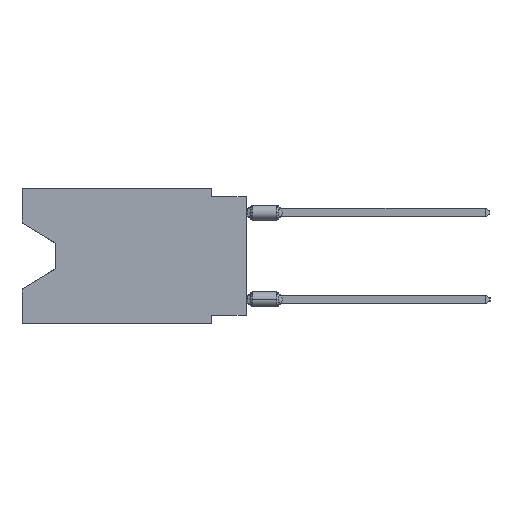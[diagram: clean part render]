
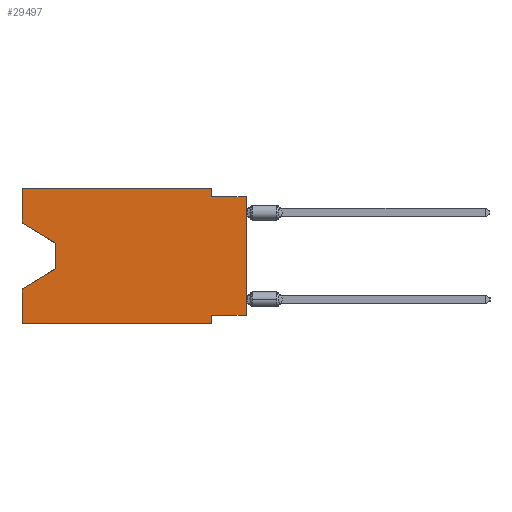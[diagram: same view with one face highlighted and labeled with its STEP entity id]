
A CAD part, left-side view. The second image highlights one B-rep face of the part: STEP entity #29497.
In plain terms, the highlighted planar face has unit normal (-1, 0, 0).
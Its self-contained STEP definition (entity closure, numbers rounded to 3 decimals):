
#1516 = CARTESIAN_POINT ( 'NONE',  ( 0., 16.383, 0. ) ) ;
#2131 = EDGE_CURVE ( 'NONE', #55517, #2793, #15696, .T. ) ;
#2134 = DIRECTION ( 'NONE',  ( 1., 0., 0. ) ) ;
#2793 = VERTEX_POINT ( 'NONE', #14090 ) ;
#3090 = CARTESIAN_POINT ( 'NONE',  ( 0., 0., -9.271 ) ) ;
#4744 = VERTEX_POINT ( 'NONE', #49859 ) ;
#5263 = VECTOR ( 'NONE', #22718, 1000. ) ;
#5686 = CARTESIAN_POINT ( 'NONE',  ( 0., 16.383, -9.906 ) ) ;
#6426 = FACE_OUTER_BOUND ( 'NONE', #46369, .T. ) ;
#6665 = EDGE_CURVE ( 'NONE', #55517, #16971, #51575, .T. ) ;
#7134 = VECTOR ( 'NONE', #56173, 1000. ) ;
#7454 = DIRECTION ( 'NONE',  ( 0., -1., 0. ) ) ;
#8672 = ORIENTED_EDGE ( 'NONE', *, *, #14410, .T. ) ;
#9556 = LINE ( 'NONE', #57363, #22292 ) ;
#12483 = VECTOR ( 'NONE', #55267, 1000. ) ;
#12492 = VECTOR ( 'NONE', #58864, 1000. ) ;
#12715 = VECTOR ( 'NONE', #55784, 1000. ) ;
#13063 = VECTOR ( 'NONE', #7454, 1000. ) ;
#13219 = CARTESIAN_POINT ( 'NONE',  ( 0., 13.97, -5.893 ) ) ;
#14090 = CARTESIAN_POINT ( 'NONE',  ( 0., 0., -0.635 ) ) ;
#14141 = DIRECTION ( 'NONE',  ( 0., 0.855, -0.519 ) ) ;
#14410 = EDGE_CURVE ( 'NONE', #4744, #47145, #36544, .T. ) ;
#15131 = CARTESIAN_POINT ( 'NONE',  ( 0., 2.54, -9.271 ) ) ;
#15696 = LINE ( 'NONE', #25502, #26946 ) ;
#16569 = VERTEX_POINT ( 'NONE', #28722 ) ;
#16971 = VERTEX_POINT ( 'NONE', #15131 ) ;
#17070 = CARTESIAN_POINT ( 'NONE',  ( 0., 16.383, 0. ) ) ;
#18372 = LINE ( 'NONE', #38292, #12715 ) ;
#19818 = EDGE_CURVE ( 'NONE', #55178, #34603, #37780, .T. ) ;
#20383 = DIRECTION ( 'NONE',  ( 0., -1., 0. ) ) ;
#20387 = ORIENTED_EDGE ( 'NONE', *, *, #24334, .T. ) ;
#20708 = VERTEX_POINT ( 'NONE', #33356 ) ;
#22292 = VECTOR ( 'NONE', #46996, 1000. ) ;
#22568 = CARTESIAN_POINT ( 'NONE',  ( 0., 2.54, 0. ) ) ;
#22718 = DIRECTION ( 'NONE',  ( 0., 0., 1. ) ) ;
#23934 = VECTOR ( 'NONE', #50823, 1000. ) ;
#24334 = EDGE_CURVE ( 'NONE', #34603, #4744, #9556, .T. ) ;
#24464 = CARTESIAN_POINT ( 'NONE',  ( 0., 16.383, -7.36 ) ) ;
#25063 = EDGE_CURVE ( 'NONE', #16569, #52150, #40426, .T. ) ;
#25502 = CARTESIAN_POINT ( 'NONE',  ( 0., 0., 0. ) ) ;
#25751 = CARTESIAN_POINT ( 'NONE',  ( 0., 2.54, 0. ) ) ;
#25879 = CARTESIAN_POINT ( 'NONE',  ( 0., 0., -0.635 ) ) ;
#26343 = EDGE_CURVE ( 'NONE', #35759, #20708, #35380, .T. ) ;
#26350 = ORIENTED_EDGE ( 'NONE', *, *, #44502, .F. ) ;
#26946 = VECTOR ( 'NONE', #39613, 1000. ) ;
#27565 = VERTEX_POINT ( 'NONE', #36009 ) ;
#27992 = EDGE_CURVE ( 'NONE', #55178, #16569, #49739, .T. ) ;
#28722 = CARTESIAN_POINT ( 'NONE',  ( 0., 16.383, 0. ) ) ;
#28999 = AXIS2_PLACEMENT_3D ( 'NONE', #1516, #2134, #39876 ) ;
#29497 = ADVANCED_FACE ( 'NONE', ( #6426 ), #53363, .F. ) ;
#29644 = ORIENTED_EDGE ( 'NONE', *, *, #25063, .F. ) ;
#31637 = CARTESIAN_POINT ( 'NONE',  ( 0., 16.383, 0. ) ) ;
#33094 = ORIENTED_EDGE ( 'NONE', *, *, #6665, .F. ) ;
#33237 = CARTESIAN_POINT ( 'NONE',  ( 0., 16.383, -2.546 ) ) ;
#33356 = CARTESIAN_POINT ( 'NONE',  ( 0., 2.54, -9.906 ) ) ;
#34196 = LINE ( 'NONE', #25879, #44272 ) ;
#34603 = VERTEX_POINT ( 'NONE', #56898 ) ;
#35252 = ORIENTED_EDGE ( 'NONE', *, *, #53370, .F. ) ;
#35380 = LINE ( 'NONE', #54088, #13063 ) ;
#35759 = VERTEX_POINT ( 'NONE', #5686 ) ;
#35805 = CARTESIAN_POINT ( 'NONE',  ( 0., 16.383, 0. ) ) ;
#36009 = CARTESIAN_POINT ( 'NONE',  ( 0., 2.54, -0.635 ) ) ;
#36544 = LINE ( 'NONE', #13219, #50545 ) ;
#36569 = CARTESIAN_POINT ( 'NONE',  ( 0., 0., -9.271 ) ) ;
#37780 = LINE ( 'NONE', #47904, #7134 ) ;
#38292 = CARTESIAN_POINT ( 'NONE',  ( 0., 2.54, -9.906 ) ) ;
#39613 = DIRECTION ( 'NONE',  ( 0., 0., 1. ) ) ;
#39876 = DIRECTION ( 'NONE',  ( 0., 0., -1. ) ) ;
#40184 = LINE ( 'NONE', #25751, #12492 ) ;
#40390 = LINE ( 'NONE', #17070, #50584 ) ;
#40426 = LINE ( 'NONE', #35805, #23934 ) ;
#42095 = EDGE_CURVE ( 'NONE', #27565, #2793, #34196, .T. ) ;
#43843 = ORIENTED_EDGE ( 'NONE', *, *, #26343, .T. ) ;
#44272 = VECTOR ( 'NONE', #20383, 1000. ) ;
#44502 = EDGE_CURVE ( 'NONE', #16971, #20708, #18372, .T. ) ;
#45295 = DIRECTION ( 'NONE',  ( 0., 0., 1. ) ) ;
#46369 = EDGE_LOOP ( 'NONE', ( #50826, #20387, #8672, #54213, #43843, #26350, #33094, #55113, #51071, #35252, #29644, #52168 ) ) ;
#46996 = DIRECTION ( 'NONE',  ( 0., 0., -1. ) ) ;
#47145 = VERTEX_POINT ( 'NONE', #24464 ) ;
#47904 = CARTESIAN_POINT ( 'NONE',  ( 0., 16.383, -2.546 ) ) ;
#49739 = LINE ( 'NONE', #31637, #5263 ) ;
#49859 = CARTESIAN_POINT ( 'NONE',  ( 0., 13.97, -5.893 ) ) ;
#50545 = VECTOR ( 'NONE', #14141, 1000. ) ;
#50584 = VECTOR ( 'NONE', #45295, 1000. ) ;
#50823 = DIRECTION ( 'NONE',  ( 0., -1., 0. ) ) ;
#50826 = ORIENTED_EDGE ( 'NONE', *, *, #19818, .T. ) ;
#51071 = ORIENTED_EDGE ( 'NONE', *, *, #42095, .F. ) ;
#51575 = LINE ( 'NONE', #36569, #12483 ) ;
#52098 = EDGE_CURVE ( 'NONE', #35759, #47145, #40390, .T. ) ;
#52150 = VERTEX_POINT ( 'NONE', #22568 ) ;
#52168 = ORIENTED_EDGE ( 'NONE', *, *, #27992, .F. ) ;
#53363 = PLANE ( 'NONE',  #28999 ) ;
#53370 = EDGE_CURVE ( 'NONE', #52150, #27565, #40184, .T. ) ;
#54088 = CARTESIAN_POINT ( 'NONE',  ( 0., 16.383, -9.906 ) ) ;
#54213 = ORIENTED_EDGE ( 'NONE', *, *, #52098, .F. ) ;
#55113 = ORIENTED_EDGE ( 'NONE', *, *, #2131, .T. ) ;
#55178 = VERTEX_POINT ( 'NONE', #33237 ) ;
#55267 = DIRECTION ( 'NONE',  ( 0., 1., 0. ) ) ;
#55517 = VERTEX_POINT ( 'NONE', #3090 ) ;
#55784 = DIRECTION ( 'NONE',  ( 0., 0., -1. ) ) ;
#56173 = DIRECTION ( 'NONE',  ( 0., -0.855, -0.519 ) ) ;
#56898 = CARTESIAN_POINT ( 'NONE',  ( 0., 13.97, -4.013 ) ) ;
#57363 = CARTESIAN_POINT ( 'NONE',  ( 0., 13.97, -4.013 ) ) ;
#58864 = DIRECTION ( 'NONE',  ( 0., 0., -1. ) ) ;
